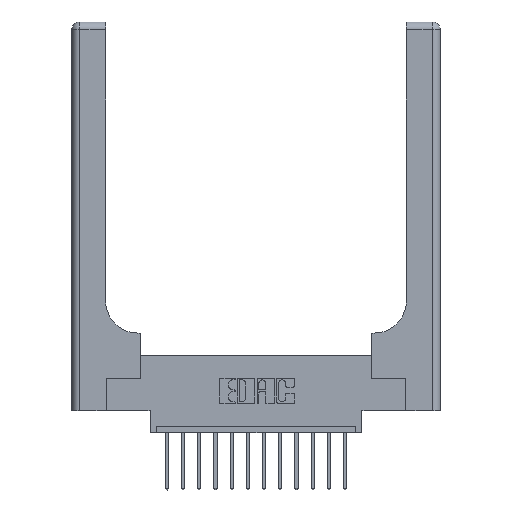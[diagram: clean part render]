
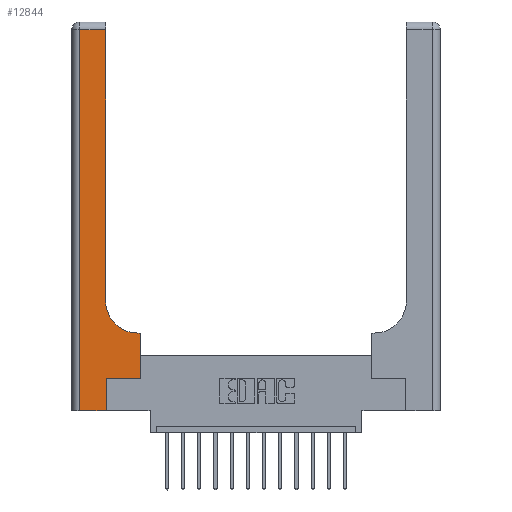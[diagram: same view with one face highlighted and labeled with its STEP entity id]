
A CAD part, top view. The second image highlights one B-rep face of the part: STEP entity #12844.
In plain terms, the highlighted planar face has unit normal (0, 0, 1).
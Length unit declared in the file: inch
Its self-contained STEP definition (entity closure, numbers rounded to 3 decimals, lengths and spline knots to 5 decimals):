
#104 = VERTEX_POINT ( 'NONE', #14543 ) ;
#503 = CARTESIAN_POINT ( 'NONE',  ( 0.528, 0.25, 0.37 ) ) ;
#627 = FACE_OUTER_BOUND ( 'NONE', #11983, .T. ) ;
#815 = VERTEX_POINT ( 'NONE', #12911 ) ;
#1361 = CARTESIAN_POINT ( 'NONE',  ( 0.06, 2.94, 0.37 ) ) ;
#1397 = EDGE_CURVE ( 'NONE', #10546, #104, #6081, .T. ) ;
#1739 = CARTESIAN_POINT ( 'NONE',  ( 0., 3., 0.37 ) ) ;
#2021 = VERTEX_POINT ( 'NONE', #15972 ) ;
#2362 = DIRECTION ( 'NONE',  ( 0., -1., 0. ) ) ;
#2510 = AXIS2_PLACEMENT_3D ( 'NONE', #9064, #13054, #7825 ) ;
#2557 = ORIENTED_EDGE ( 'NONE', *, *, #8854, .T. ) ;
#2672 = ORIENTED_EDGE ( 'NONE', *, *, #10093, .T. ) ;
#2773 = DIRECTION ( 'NONE',  ( 1., 0., 0. ) ) ;
#3297 = DIRECTION ( 'NONE',  ( 0., 1., 0. ) ) ;
#3421 = VERTEX_POINT ( 'NONE', #16145 ) ;
#3692 = DIRECTION ( 'NONE',  ( 0., 1., 0. ) ) ;
#4202 = VERTEX_POINT ( 'NONE', #503 ) ;
#4246 = ORIENTED_EDGE ( 'NONE', *, *, #1397, .T. ) ;
#5197 = LINE ( 'NONE', #14094, #8264 ) ;
#5271 = DIRECTION ( 'NONE',  ( -1., 0., 0. ) ) ;
#5754 = VECTOR ( 'NONE', #16428, 39.37008 ) ;
#5896 = EDGE_CURVE ( 'NONE', #104, #16233, #7170, .T. ) ;
#5950 = CARTESIAN_POINT ( 'NONE',  ( 0.528, 0.25, 0.37 ) ) ;
#6081 = LINE ( 'NONE', #11461, #7319 ) ;
#6198 = LINE ( 'NONE', #5950, #6613 ) ;
#6382 = EDGE_CURVE ( 'NONE', #16233, #815, #6974, .T. ) ;
#6533 = LINE ( 'NONE', #16608, #11210 ) ;
#6613 = VECTOR ( 'NONE', #3297, 39.37008 ) ;
#6703 = EDGE_CURVE ( 'NONE', #6792, #14715, #6533, .T. ) ;
#6792 = VERTEX_POINT ( 'NONE', #8396 ) ;
#6961 = CARTESIAN_POINT ( 'NONE',  ( 0.265, 0., 0.37 ) ) ;
#6974 = LINE ( 'NONE', #10273, #13829 ) ;
#7170 = LINE ( 'NONE', #12600, #5754 ) ;
#7197 = ORIENTED_EDGE ( 'NONE', *, *, #14283, .T. ) ;
#7222 = EDGE_CURVE ( 'NONE', #3421, #2021, #15221, .T. ) ;
#7319 = VECTOR ( 'NONE', #3692, 39.37008 ) ;
#7825 = DIRECTION ( 'NONE',  ( 1., 0., 0. ) ) ;
#7871 = LINE ( 'NONE', #8698, #13726 ) ;
#8053 = ORIENTED_EDGE ( 'NONE', *, *, #7222, .T. ) ;
#8244 = ORIENTED_EDGE ( 'NONE', *, *, #6382, .T. ) ;
#8264 = VECTOR ( 'NONE', #2773, 39.37008 ) ;
#8396 = CARTESIAN_POINT ( 'NONE',  ( 0.528, 0.6, 0.37 ) ) ;
#8618 = CARTESIAN_POINT ( 'NONE',  ( 0.26, 0.85, 0.37 ) ) ;
#8687 = CIRCLE ( 'NONE', #2510, 0.25 ) ;
#8698 = CARTESIAN_POINT ( 'NONE',  ( 0., 0., 0.37 ) ) ;
#8854 = EDGE_CURVE ( 'NONE', #815, #3421, #7871, .T. ) ;
#9064 = CARTESIAN_POINT ( 'NONE',  ( 0.51, 0.85, 0.37 ) ) ;
#9189 = EDGE_CURVE ( 'NONE', #2021, #4202, #5197, .T. ) ;
#9396 = AXIS2_PLACEMENT_3D ( 'NONE', #1739, #9455, #15850 ) ;
#9455 = DIRECTION ( 'NONE',  ( 0., 0., -1. ) ) ;
#10093 = EDGE_CURVE ( 'NONE', #4202, #6792, #6198, .T. ) ;
#10273 = CARTESIAN_POINT ( 'NONE',  ( 0.06, 3., 0.37 ) ) ;
#10546 = VERTEX_POINT ( 'NONE', #8618 ) ;
#10803 = PLANE ( 'NONE',  #9396 ) ;
#10880 = ORIENTED_EDGE ( 'NONE', *, *, #6703, .T. ) ;
#11210 = VECTOR ( 'NONE', #5271, 39.37008 ) ;
#11262 = CARTESIAN_POINT ( 'NONE',  ( 0.51, 0.6, 0.37 ) ) ;
#11461 = CARTESIAN_POINT ( 'NONE',  ( 0.26, 3., 0.37 ) ) ;
#11684 = ORIENTED_EDGE ( 'NONE', *, *, #5896, .T. ) ;
#11983 = EDGE_LOOP ( 'NONE', ( #4246, #11684, #8244, #2557, #8053, #13776, #2672, #10880, #7197 ) ) ;
#12600 = CARTESIAN_POINT ( 'NONE',  ( 0., 2.94, 0.37 ) ) ;
#12844 = ADVANCED_FACE ( 'NONE', ( #627 ), #10803, .F. ) ;
#12911 = CARTESIAN_POINT ( 'NONE',  ( 0.06, 0., 0.37 ) ) ;
#13054 = DIRECTION ( 'NONE',  ( 0., 0., -1. ) ) ;
#13726 = VECTOR ( 'NONE', #16513, 39.37008 ) ;
#13776 = ORIENTED_EDGE ( 'NONE', *, *, #9189, .T. ) ;
#13829 = VECTOR ( 'NONE', #2362, 39.37008 ) ;
#14094 = CARTESIAN_POINT ( 'NONE',  ( 0.265, 0.25, 0.37 ) ) ;
#14283 = EDGE_CURVE ( 'NONE', #14715, #10546, #8687, .T. ) ;
#14543 = CARTESIAN_POINT ( 'NONE',  ( 0.26, 2.94, 0.37 ) ) ;
#14579 = DIRECTION ( 'NONE',  ( 0., 1., 0. ) ) ;
#14715 = VERTEX_POINT ( 'NONE', #11262 ) ;
#15221 = LINE ( 'NONE', #6961, #15223 ) ;
#15223 = VECTOR ( 'NONE', #14579, 39.37008 ) ;
#15850 = DIRECTION ( 'NONE',  ( -1., 0., 0. ) ) ;
#15972 = CARTESIAN_POINT ( 'NONE',  ( 0.265, 0.25, 0.37 ) ) ;
#16145 = CARTESIAN_POINT ( 'NONE',  ( 0.265, 0., 0.37 ) ) ;
#16233 = VERTEX_POINT ( 'NONE', #1361 ) ;
#16428 = DIRECTION ( 'NONE',  ( -1., 0., 0. ) ) ;
#16513 = DIRECTION ( 'NONE',  ( 1., 0., 0. ) ) ;
#16608 = CARTESIAN_POINT ( 'NONE',  ( 0.26, 0.6, 0.37 ) ) ;
